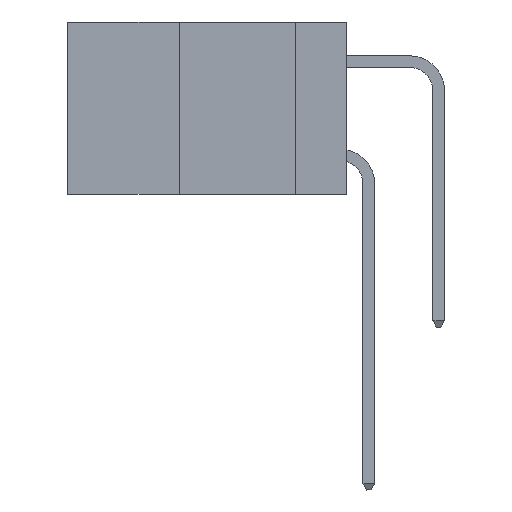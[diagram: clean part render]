
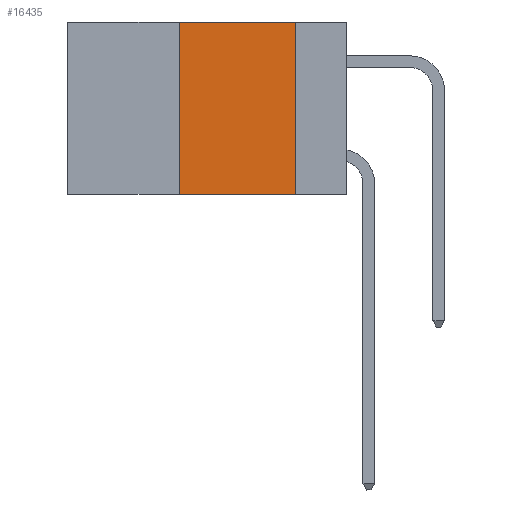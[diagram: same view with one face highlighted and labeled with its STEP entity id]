
A CAD part, left-side view. The second image highlights one B-rep face of the part: STEP entity #16435.
In plain terms, the highlighted planar face has unit normal (-1, 0, 0).
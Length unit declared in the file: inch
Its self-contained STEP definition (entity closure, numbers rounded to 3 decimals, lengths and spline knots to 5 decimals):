
#272 = DIRECTION ( 'NONE',  ( 1., 0., 0. ) ) ;
#420 = EDGE_LOOP ( 'NONE', ( #16489, #15317, #3376, #10337 ) ) ;
#1458 = CARTESIAN_POINT ( 'NONE',  ( 0., 0.36, 0. ) ) ;
#1553 = CARTESIAN_POINT ( 'NONE',  ( 0., 0.6, 0. ) ) ;
#1775 = DIRECTION ( 'NONE',  ( 0., -1., 0. ) ) ;
#1825 = VECTOR ( 'NONE', #2672, 39.37008 ) ;
#2672 = DIRECTION ( 'NONE',  ( 0., -1., 0. ) ) ;
#2835 = CARTESIAN_POINT ( 'NONE',  ( 0., 0.6, 0. ) ) ;
#2929 = VECTOR ( 'NONE', #12108, 39.37008 ) ;
#3376 = ORIENTED_EDGE ( 'NONE', *, *, #4414, .F. ) ;
#3481 = CARTESIAN_POINT ( 'NONE',  ( 0., 0.11, 0. ) ) ;
#3568 = CARTESIAN_POINT ( 'NONE',  ( 0., 0.36, -0.37 ) ) ;
#3620 = VERTEX_POINT ( 'NONE', #3568 ) ;
#4260 = CARTESIAN_POINT ( 'NONE',  ( 0., 0.6, -0.37 ) ) ;
#4344 = LINE ( 'NONE', #7045, #2929 ) ;
#4414 = EDGE_CURVE ( 'NONE', #3620, #4792, #4344, .T. ) ;
#4417 = CARTESIAN_POINT ( 'NONE',  ( 0., 0.11, 0. ) ) ;
#4787 = DIRECTION ( 'NONE',  ( 0., 0., -1. ) ) ;
#4792 = VERTEX_POINT ( 'NONE', #1458 ) ;
#6508 = LINE ( 'NONE', #4260, #16188 ) ;
#6801 = VERTEX_POINT ( 'NONE', #12790 ) ;
#6961 = AXIS2_PLACEMENT_3D ( 'NONE', #1553, #272, #10835 ) ;
#7045 = CARTESIAN_POINT ( 'NONE',  ( 0., 0.36, 0. ) ) ;
#9491 = EDGE_CURVE ( 'NONE', #12149, #6801, #9967, .T. ) ;
#9967 = LINE ( 'NONE', #3481, #15132 ) ;
#10070 = LINE ( 'NONE', #2835, #1825 ) ;
#10337 = ORIENTED_EDGE ( 'NONE', *, *, #16007, .T. ) ;
#10835 = DIRECTION ( 'NONE',  ( 0., 0., -1. ) ) ;
#12108 = DIRECTION ( 'NONE',  ( 0., 0., 1. ) ) ;
#12149 = VERTEX_POINT ( 'NONE', #4417 ) ;
#12790 = CARTESIAN_POINT ( 'NONE',  ( 0., 0.11, -0.37 ) ) ;
#14184 = EDGE_CURVE ( 'NONE', #4792, #12149, #10070, .T. ) ;
#14359 = FACE_OUTER_BOUND ( 'NONE', #420, .T. ) ;
#15132 = VECTOR ( 'NONE', #4787, 39.37008 ) ;
#15317 = ORIENTED_EDGE ( 'NONE', *, *, #14184, .F. ) ;
#16007 = EDGE_CURVE ( 'NONE', #3620, #6801, #6508, .T. ) ;
#16024 = PLANE ( 'NONE',  #6961 ) ;
#16188 = VECTOR ( 'NONE', #1775, 39.37008 ) ;
#16435 = ADVANCED_FACE ( 'NONE', ( #14359 ), #16024, .F. ) ;
#16489 = ORIENTED_EDGE ( 'NONE', *, *, #9491, .F. ) ;
